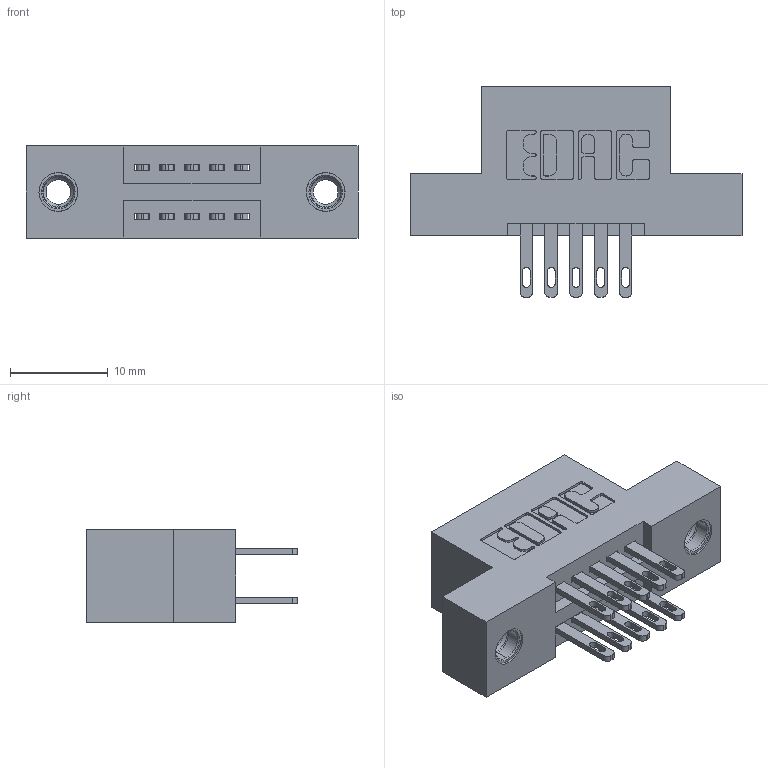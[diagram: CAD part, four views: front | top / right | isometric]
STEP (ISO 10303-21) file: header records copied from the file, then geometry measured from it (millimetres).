
FILE_DESCRIPTION (( 'STEP AP203' ), '1' );
FILE_NAME ('345-010-500-207.STEP', '2018-08-17T07:33:52', ( '' ), ( '' ), 'SwSTEP 2.0', 'SolidWorks 2016', '' );
FILE_SCHEMA (( 'CONFIG_CONTROL_DESIGN' ));
Length unit declared in the file: inch
Products named in the file (4): 345 Part_Flush Mounting Lugs - 0.156 Dia-TI; 345-292-001_345-293-100; 345-250-001_345-250-005-103; 345-010-500-207
Assembly tree (13 placements, depth 2):
  345-010-500-207
    345 Part_Flush Mounting Lugs - 0.156 Dia-TI
    345-292-001_345-293-100  x10
    345-250-001_345-250-005-103  x2
Bounding box: 33.91 x 21.51 x 9.4 mm (x, y, z)
Volume: 2967.5 mm3; surface area: 3799.8 mm2
Topology: 13 solids, 13 shells, 646 faces, 1887 edges, 1250 vertices
Faces by surface type: plane 382, cylinder 248, cone 12, torus 4
Entity records: 10020 total; most frequent: CARTESIAN_POINT 1695, ORIENTED_EDGE 1622, DIRECTION 1569, EDGE_CURVE 811, VECTOR 635, LINE 635, VERTEX_POINT 536, AXIS2_PLACEMENT_3D 467
